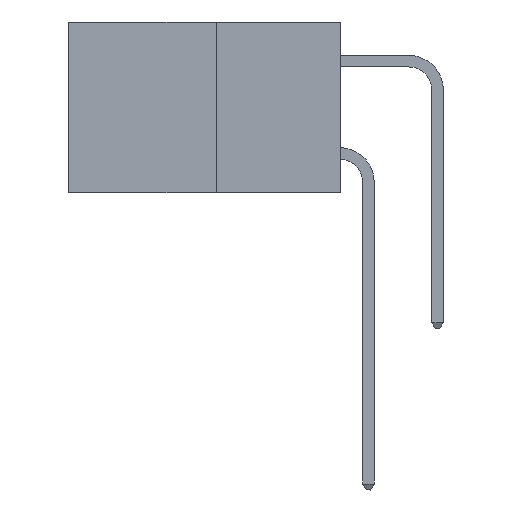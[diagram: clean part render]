
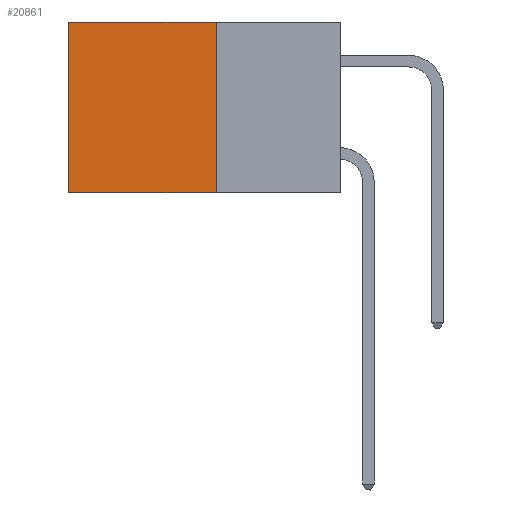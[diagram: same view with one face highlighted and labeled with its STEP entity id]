
A CAD part, left-side view. The second image highlights one B-rep face of the part: STEP entity #20861.
In plain terms, the highlighted planar face has unit normal (-1, 0, 0).
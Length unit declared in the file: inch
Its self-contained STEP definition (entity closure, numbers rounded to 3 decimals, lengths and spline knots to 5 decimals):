
#334 = ORIENTED_EDGE ( 'NONE', *, *, #13783, .F. ) ;
#1333 = CARTESIAN_POINT ( 'NONE',  ( 0.277, 0.27, -0.37 ) ) ;
#1581 = FACE_OUTER_BOUND ( 'NONE', #10730, .T. ) ;
#2459 = PLANE ( 'NONE',  #11731 ) ;
#2854 = EDGE_CURVE ( 'NONE', #5725, #9133, #25636, .T. ) ;
#3745 = LINE ( 'NONE', #26506, #14534 ) ;
#4094 = EDGE_CURVE ( 'NONE', #18270, #4284, #18136, .T. ) ;
#4284 = VERTEX_POINT ( 'NONE', #9639 ) ;
#4981 = DIRECTION ( 'NONE',  ( 0., 0., -1. ) ) ;
#5725 = VERTEX_POINT ( 'NONE', #1333 ) ;
#6792 = VECTOR ( 'NONE', #21959, 39.37008 ) ;
#6882 = CARTESIAN_POINT ( 'NONE',  ( 0.277, 0.27, -0.37 ) ) ;
#7485 = LINE ( 'NONE', #11555, #8829 ) ;
#7874 = ORIENTED_EDGE ( 'NONE', *, *, #14283, .T. ) ;
#8704 = CARTESIAN_POINT ( 'NONE',  ( 0.277, 0.27, 0. ) ) ;
#8829 = VECTOR ( 'NONE', #26582, 39.37008 ) ;
#9057 = DIRECTION ( 'NONE',  ( 0., 0., -1. ) ) ;
#9091 = ORIENTED_EDGE ( 'NONE', *, *, #4094, .T. ) ;
#9133 = VERTEX_POINT ( 'NONE', #18959 ) ;
#9639 = CARTESIAN_POINT ( 'NONE',  ( 0.277, 0.59, 0. ) ) ;
#10730 = EDGE_LOOP ( 'NONE', ( #7874, #13656, #334, #9091 ) ) ;
#11555 = CARTESIAN_POINT ( 'NONE',  ( 0.277, 0.59, -0.37 ) ) ;
#11731 = AXIS2_PLACEMENT_3D ( 'NONE', #6882, #21824, #9057 ) ;
#13656 = ORIENTED_EDGE ( 'NONE', *, *, #2854, .F. ) ;
#13783 = EDGE_CURVE ( 'NONE', #18270, #5725, #3745, .T. ) ;
#14233 = VECTOR ( 'NONE', #25007, 39.37008 ) ;
#14283 = EDGE_CURVE ( 'NONE', #4284, #9133, #7485, .T. ) ;
#14534 = VECTOR ( 'NONE', #4981, 39.37008 ) ;
#18136 = LINE ( 'NONE', #26126, #6792 ) ;
#18270 = VERTEX_POINT ( 'NONE', #8704 ) ;
#18959 = CARTESIAN_POINT ( 'NONE',  ( 0.277, 0.59, -0.37 ) ) ;
#20861 = ADVANCED_FACE ( 'NONE', ( #1581 ), #2459, .F. ) ;
#21824 = DIRECTION ( 'NONE',  ( 1., 0., 0. ) ) ;
#21959 = DIRECTION ( 'NONE',  ( 0., 1., 0. ) ) ;
#22747 = CARTESIAN_POINT ( 'NONE',  ( 0.277, 0.27, -0.37 ) ) ;
#25007 = DIRECTION ( 'NONE',  ( 0., 1., 0. ) ) ;
#25636 = LINE ( 'NONE', #22747, #14233 ) ;
#26126 = CARTESIAN_POINT ( 'NONE',  ( 0.277, 0.27, 0. ) ) ;
#26506 = CARTESIAN_POINT ( 'NONE',  ( 0.277, 0.27, -0.37 ) ) ;
#26582 = DIRECTION ( 'NONE',  ( 0., 0., -1. ) ) ;
